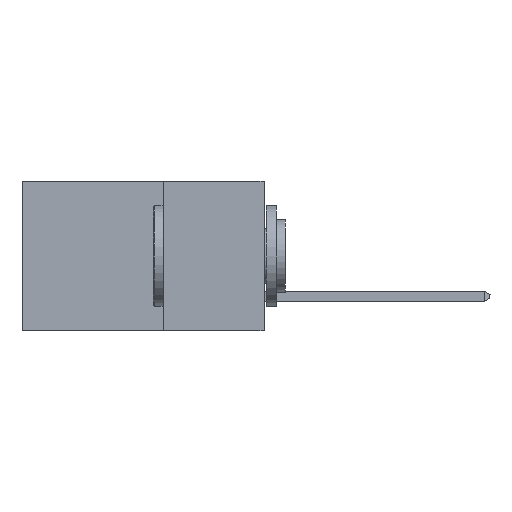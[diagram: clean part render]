
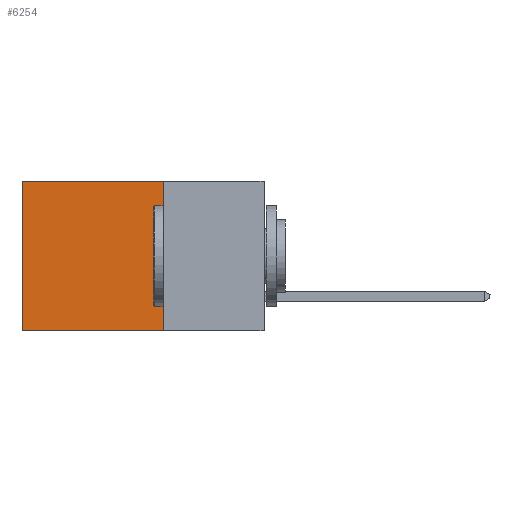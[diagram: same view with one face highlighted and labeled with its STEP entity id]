
A CAD part, left-side view. The second image highlights one B-rep face of the part: STEP entity #6254.
In plain terms, the highlighted planar face has unit normal (-1, 0, 0).
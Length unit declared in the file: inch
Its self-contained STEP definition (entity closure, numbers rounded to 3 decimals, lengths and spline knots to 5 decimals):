
#500 = EDGE_CURVE ( 'NONE', #2047, #647, #5702, .T. ) ;
#647 = VERTEX_POINT ( 'NONE', #14055 ) ;
#2047 = VERTEX_POINT ( 'NONE', #5027 ) ;
#3518 = VECTOR ( 'NONE', #11964, 39.37008 ) ;
#3609 = CARTESIAN_POINT ( 'NONE',  ( 0.2615, 0.25, -0.37 ) ) ;
#4362 = EDGE_CURVE ( 'NONE', #13266, #647, #8421, .T. ) ;
#4657 = FACE_OUTER_BOUND ( 'NONE', #17435, .T. ) ;
#4764 = DIRECTION ( 'NONE',  ( 1., 0., 0. ) ) ;
#4797 = VERTEX_POINT ( 'NONE', #15398 ) ;
#5027 = CARTESIAN_POINT ( 'NONE',  ( 0.2615, 0.6, 0. ) ) ;
#5340 = ORIENTED_EDGE ( 'NONE', *, *, #500, .T. ) ;
#5390 = AXIS2_PLACEMENT_3D ( 'NONE', #11461, #4764, #18245 ) ;
#5702 = LINE ( 'NONE', #8942, #16842 ) ;
#5730 = EDGE_CURVE ( 'NONE', #4797, #13266, #17096, .T. ) ;
#5832 = CARTESIAN_POINT ( 'NONE',  ( 0.2615, 0.25, -0.37 ) ) ;
#6254 = ADVANCED_FACE ( 'NONE', ( #4657 ), #21582, .F. ) ;
#6780 = CARTESIAN_POINT ( 'NONE',  ( 0.2615, 0.25, 0. ) ) ;
#8421 = LINE ( 'NONE', #3609, #3518 ) ;
#8942 = CARTESIAN_POINT ( 'NONE',  ( 0.2615, 0.6, -0.37 ) ) ;
#11459 = DIRECTION ( 'NONE',  ( 0., 1., 0. ) ) ;
#11461 = CARTESIAN_POINT ( 'NONE',  ( 0.2615, 0.25, -0.37 ) ) ;
#11964 = DIRECTION ( 'NONE',  ( 0., 1., 0. ) ) ;
#12237 = ORIENTED_EDGE ( 'NONE', *, *, #19575, .T. ) ;
#13266 = VERTEX_POINT ( 'NONE', #5832 ) ;
#13551 = CARTESIAN_POINT ( 'NONE',  ( 0.2615, 0.25, -0.37 ) ) ;
#13661 = ORIENTED_EDGE ( 'NONE', *, *, #4362, .F. ) ;
#14055 = CARTESIAN_POINT ( 'NONE',  ( 0.2615, 0.6, -0.37 ) ) ;
#15398 = CARTESIAN_POINT ( 'NONE',  ( 0.2615, 0.25, 0. ) ) ;
#16842 = VECTOR ( 'NONE', #18835, 39.37008 ) ;
#16981 = DIRECTION ( 'NONE',  ( 0., 0., -1. ) ) ;
#17096 = LINE ( 'NONE', #13551, #19585 ) ;
#17435 = EDGE_LOOP ( 'NONE', ( #5340, #13661, #17798, #12237 ) ) ;
#17798 = ORIENTED_EDGE ( 'NONE', *, *, #5730, .F. ) ;
#18245 = DIRECTION ( 'NONE',  ( 0., 0., -1. ) ) ;
#18676 = LINE ( 'NONE', #6780, #19854 ) ;
#18835 = DIRECTION ( 'NONE',  ( 0., 0., -1. ) ) ;
#19575 = EDGE_CURVE ( 'NONE', #4797, #2047, #18676, .T. ) ;
#19585 = VECTOR ( 'NONE', #16981, 39.37008 ) ;
#19854 = VECTOR ( 'NONE', #11459, 39.37008 ) ;
#21582 = PLANE ( 'NONE',  #5390 ) ;
